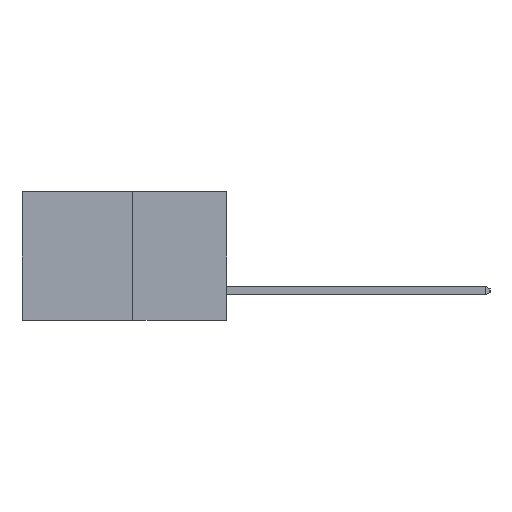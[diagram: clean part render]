
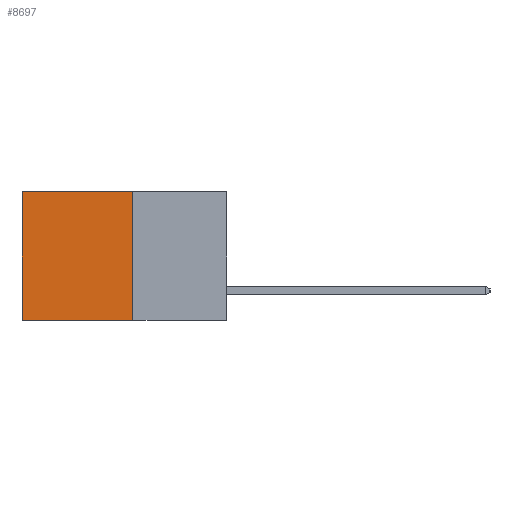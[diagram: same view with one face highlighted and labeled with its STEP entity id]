
A CAD part, left-side view. The second image highlights one B-rep face of the part: STEP entity #8697.
In plain terms, the highlighted planar face has unit normal (-1, 0, 0).
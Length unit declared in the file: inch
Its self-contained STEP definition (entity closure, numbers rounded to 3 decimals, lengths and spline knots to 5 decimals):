
#870 = FACE_OUTER_BOUND ( 'NONE', #6025, .T. ) ;
#1207 = EDGE_CURVE ( 'NONE', #2614, #4656, #12156, .T. ) ;
#1360 = CARTESIAN_POINT ( 'NONE',  ( 0.277, 0.27, -0.37 ) ) ;
#1399 = CARTESIAN_POINT ( 'NONE',  ( 0.277, 0.27, -0.37 ) ) ;
#2048 = VECTOR ( 'NONE', #2430, 39.37008 ) ;
#2430 = DIRECTION ( 'NONE',  ( 0., 1., 0. ) ) ;
#2614 = VERTEX_POINT ( 'NONE', #11612 ) ;
#2762 = VERTEX_POINT ( 'NONE', #12643 ) ;
#3212 = DIRECTION ( 'NONE',  ( 0., 0., -1. ) ) ;
#3239 = ORIENTED_EDGE ( 'NONE', *, *, #8393, .F. ) ;
#3394 = VERTEX_POINT ( 'NONE', #6252 ) ;
#4201 = ORIENTED_EDGE ( 'NONE', *, *, #1207, .F. ) ;
#4531 = DIRECTION ( 'NONE',  ( 0., 0., -1. ) ) ;
#4656 = VERTEX_POINT ( 'NONE', #5843 ) ;
#4926 = DIRECTION ( 'NONE',  ( 0., 1., 0. ) ) ;
#5153 = ORIENTED_EDGE ( 'NONE', *, *, #10422, .T. ) ;
#5482 = ORIENTED_EDGE ( 'NONE', *, *, #9179, .T. ) ;
#5766 = VECTOR ( 'NONE', #11839, 39.37008 ) ;
#5843 = CARTESIAN_POINT ( 'NONE',  ( 0.277, 0.27, -0.37 ) ) ;
#6025 = EDGE_LOOP ( 'NONE', ( #5482, #3239, #4201, #5153 ) ) ;
#6252 = CARTESIAN_POINT ( 'NONE',  ( 0.277, 0.59, 0. ) ) ;
#6882 = VECTOR ( 'NONE', #4531, 39.37008 ) ;
#8215 = CARTESIAN_POINT ( 'NONE',  ( 0.277, 0.27, -0.37 ) ) ;
#8393 = EDGE_CURVE ( 'NONE', #4656, #2762, #12409, .T. ) ;
#8697 = ADVANCED_FACE ( 'NONE', ( #870 ), #9188, .F. ) ;
#9005 = LINE ( 'NONE', #12788, #11300 ) ;
#9179 = EDGE_CURVE ( 'NONE', #3394, #2762, #11634, .T. ) ;
#9188 = PLANE ( 'NONE',  #9606 ) ;
#9240 = DIRECTION ( 'NONE',  ( 1., 0., 0. ) ) ;
#9606 = AXIS2_PLACEMENT_3D ( 'NONE', #8215, #9240, #3212 ) ;
#10422 = EDGE_CURVE ( 'NONE', #2614, #3394, #9005, .T. ) ;
#10893 = CARTESIAN_POINT ( 'NONE',  ( 0.277, 0.59, -0.37 ) ) ;
#11300 = VECTOR ( 'NONE', #4926, 39.37008 ) ;
#11612 = CARTESIAN_POINT ( 'NONE',  ( 0.277, 0.27, 0. ) ) ;
#11634 = LINE ( 'NONE', #10893, #5766 ) ;
#11839 = DIRECTION ( 'NONE',  ( 0., 0., -1. ) ) ;
#12156 = LINE ( 'NONE', #1399, #6882 ) ;
#12409 = LINE ( 'NONE', #1360, #2048 ) ;
#12643 = CARTESIAN_POINT ( 'NONE',  ( 0.277, 0.59, -0.37 ) ) ;
#12788 = CARTESIAN_POINT ( 'NONE',  ( 0.277, 0.27, 0. ) ) ;
